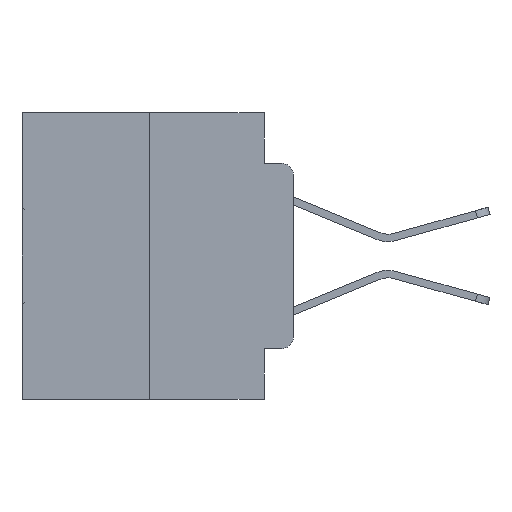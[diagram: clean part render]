
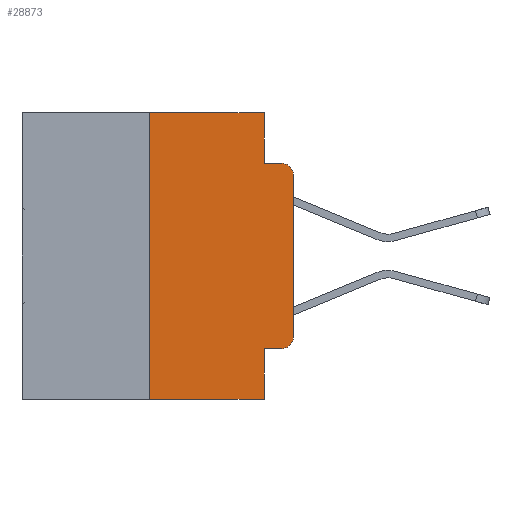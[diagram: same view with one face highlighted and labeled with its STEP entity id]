
A CAD part, left-side view. The second image highlights one B-rep face of the part: STEP entity #28873.
In plain terms, the highlighted planar face has unit normal (-1, 0, 0).
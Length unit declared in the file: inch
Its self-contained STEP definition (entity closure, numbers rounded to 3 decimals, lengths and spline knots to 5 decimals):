
#455 = LINE ( 'NONE', #28708, #25226 ) ;
#846 = CARTESIAN_POINT ( 'NONE',  ( 0., 0.473, -0.5 ) ) ;
#942 = CARTESIAN_POINT ( 'NONE',  ( 0., 0.051, -0.4115 ) ) ;
#1026 = VECTOR ( 'NONE', #17791, 39.37008 ) ;
#1735 = EDGE_CURVE ( 'NONE', #5797, #27062, #6326, .T. ) ;
#1969 = ORIENTED_EDGE ( 'NONE', *, *, #2559, .T. ) ;
#1998 = VERTEX_POINT ( 'NONE', #24383 ) ;
#2559 = EDGE_CURVE ( 'NONE', #25242, #21102, #18597, .T. ) ;
#2735 = CARTESIAN_POINT ( 'NONE',  ( 0., 0.25, 0. ) ) ;
#2850 = VECTOR ( 'NONE', #8348, 39.37008 ) ;
#3071 = LINE ( 'NONE', #30133, #22163 ) ;
#3490 = DIRECTION ( 'NONE',  ( 0., -1., 0. ) ) ;
#4725 = CIRCLE ( 'NONE', #7302, 0.02 ) ;
#5437 = ORIENTED_EDGE ( 'NONE', *, *, #1735, .F. ) ;
#5797 = VERTEX_POINT ( 'NONE', #2735 ) ;
#5911 = PLANE ( 'NONE',  #24467 ) ;
#6326 = LINE ( 'NONE', #21252, #30775 ) ;
#6541 = DIRECTION ( 'NONE',  ( -1., 0., 0. ) ) ;
#6885 = LINE ( 'NONE', #846, #1026 ) ;
#6952 = EDGE_CURVE ( 'NONE', #25242, #12352, #15697, .T. ) ;
#7302 = AXIS2_PLACEMENT_3D ( 'NONE', #13841, #30273, #16200 ) ;
#8348 = DIRECTION ( 'NONE',  ( 0., 0., -1. ) ) ;
#8374 = CARTESIAN_POINT ( 'NONE',  ( 0., 0.473, 0. ) ) ;
#9539 = DIRECTION ( 'NONE',  ( 0., 0., 1. ) ) ;
#9930 = LINE ( 'NONE', #14345, #21464 ) ;
#10617 = CARTESIAN_POINT ( 'NONE',  ( 0., 0.051, 0. ) ) ;
#10643 = CARTESIAN_POINT ( 'NONE',  ( 0., 0.051, 0. ) ) ;
#10770 = DIRECTION ( 'NONE',  ( 0., 0., -1. ) ) ;
#11891 = VERTEX_POINT ( 'NONE', #21829 ) ;
#12352 = VERTEX_POINT ( 'NONE', #16467 ) ;
#12654 = ORIENTED_EDGE ( 'NONE', *, *, #6952, .F. ) ;
#12931 = LINE ( 'NONE', #13144, #18455 ) ;
#13144 = CARTESIAN_POINT ( 'NONE',  ( 0., 0.051, -0.0885 ) ) ;
#13380 = EDGE_CURVE ( 'NONE', #1998, #5797, #9930, .T. ) ;
#13678 = ORIENTED_EDGE ( 'NONE', *, *, #14377, .F. ) ;
#13720 = CARTESIAN_POINT ( 'NONE',  ( 0., 0.02, -0.0885 ) ) ;
#13784 = EDGE_CURVE ( 'NONE', #11891, #30010, #3071, .T. ) ;
#13841 = CARTESIAN_POINT ( 'NONE',  ( 0., 0.02, -0.1085 ) ) ;
#14345 = CARTESIAN_POINT ( 'NONE',  ( 0., 0.25, 0. ) ) ;
#14377 = EDGE_CURVE ( 'NONE', #27418, #21012, #12931, .T. ) ;
#14622 = DIRECTION ( 'NONE',  ( 0., 0., -1. ) ) ;
#15613 = AXIS2_PLACEMENT_3D ( 'NONE', #20792, #6541, #23132 ) ;
#15697 = LINE ( 'NONE', #10643, #2850 ) ;
#16050 = DIRECTION ( 'NONE',  ( 0., 0., 1. ) ) ;
#16200 = DIRECTION ( 'NONE',  ( 0., 0., -1. ) ) ;
#16223 = ORIENTED_EDGE ( 'NONE', *, *, #13784, .T. ) ;
#16467 = CARTESIAN_POINT ( 'NONE',  ( 0., 0.051, -0.5 ) ) ;
#17065 = EDGE_LOOP ( 'NONE', ( #16223, #22470, #13678, #27298, #5437, #19642, #23317, #12654, #1969, #17112 ) ) ;
#17112 = ORIENTED_EDGE ( 'NONE', *, *, #17718, .T. ) ;
#17718 = EDGE_CURVE ( 'NONE', #21102, #11891, #26530, .T. ) ;
#17791 = DIRECTION ( 'NONE',  ( 0., -1., 0. ) ) ;
#18145 = EDGE_CURVE ( 'NONE', #1998, #12352, #6885, .T. ) ;
#18455 = VECTOR ( 'NONE', #3490, 39.37008 ) ;
#18597 = LINE ( 'NONE', #23910, #20075 ) ;
#19642 = ORIENTED_EDGE ( 'NONE', *, *, #13380, .F. ) ;
#20075 = VECTOR ( 'NONE', #23946, 39.37008 ) ;
#20792 = CARTESIAN_POINT ( 'NONE',  ( 0., 0.02, -0.3915 ) ) ;
#20996 = DIRECTION ( 'NONE',  ( 0., -1., 0. ) ) ;
#21012 = VERTEX_POINT ( 'NONE', #13720 ) ;
#21102 = VERTEX_POINT ( 'NONE', #23477 ) ;
#21252 = CARTESIAN_POINT ( 'NONE',  ( 0., 0.473, 0. ) ) ;
#21261 = EDGE_CURVE ( 'NONE', #27062, #27418, #455, .T. ) ;
#21464 = VECTOR ( 'NONE', #9539, 39.37008 ) ;
#21829 = CARTESIAN_POINT ( 'NONE',  ( 0., 0., -0.3915 ) ) ;
#22163 = VECTOR ( 'NONE', #16050, 39.37008 ) ;
#22246 = EDGE_CURVE ( 'NONE', #30010, #21012, #4725, .T. ) ;
#22470 = ORIENTED_EDGE ( 'NONE', *, *, #22246, .T. ) ;
#23132 = DIRECTION ( 'NONE',  ( 0., 0., -1. ) ) ;
#23317 = ORIENTED_EDGE ( 'NONE', *, *, #18145, .T. ) ;
#23477 = CARTESIAN_POINT ( 'NONE',  ( 0., 0.02, -0.4115 ) ) ;
#23910 = CARTESIAN_POINT ( 'NONE',  ( 0., 0.051, -0.4115 ) ) ;
#23946 = DIRECTION ( 'NONE',  ( 0., -1., 0. ) ) ;
#24375 = FACE_OUTER_BOUND ( 'NONE', #17065, .T. ) ;
#24383 = CARTESIAN_POINT ( 'NONE',  ( 0., 0.25, -0.5 ) ) ;
#24467 = AXIS2_PLACEMENT_3D ( 'NONE', #8374, #24892, #10770 ) ;
#24892 = DIRECTION ( 'NONE',  ( 1., 0., 0. ) ) ;
#24929 = CARTESIAN_POINT ( 'NONE',  ( 0., 0., -0.1085 ) ) ;
#25226 = VECTOR ( 'NONE', #14622, 39.37008 ) ;
#25242 = VERTEX_POINT ( 'NONE', #942 ) ;
#26530 = CIRCLE ( 'NONE', #15613, 0.02 ) ;
#27062 = VERTEX_POINT ( 'NONE', #10617 ) ;
#27298 = ORIENTED_EDGE ( 'NONE', *, *, #21261, .F. ) ;
#27418 = VERTEX_POINT ( 'NONE', #29098 ) ;
#28708 = CARTESIAN_POINT ( 'NONE',  ( 0., 0.051, 0. ) ) ;
#28873 = ADVANCED_FACE ( 'NONE', ( #24375 ), #5911, .F. ) ;
#29098 = CARTESIAN_POINT ( 'NONE',  ( 0., 0.051, -0.0885 ) ) ;
#30010 = VERTEX_POINT ( 'NONE', #24929 ) ;
#30133 = CARTESIAN_POINT ( 'NONE',  ( 0., 0., 0. ) ) ;
#30273 = DIRECTION ( 'NONE',  ( -1., 0., 0. ) ) ;
#30775 = VECTOR ( 'NONE', #20996, 39.37008 ) ;
